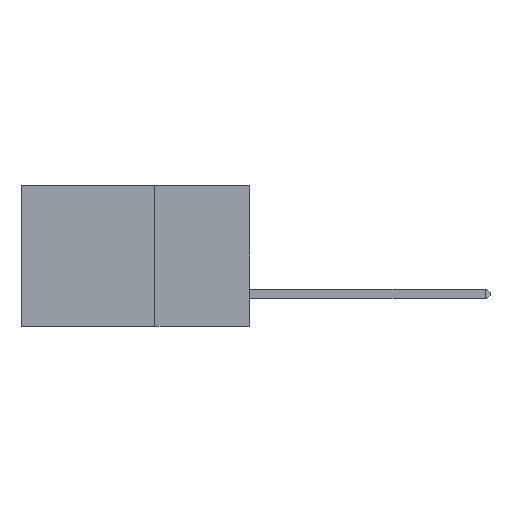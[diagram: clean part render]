
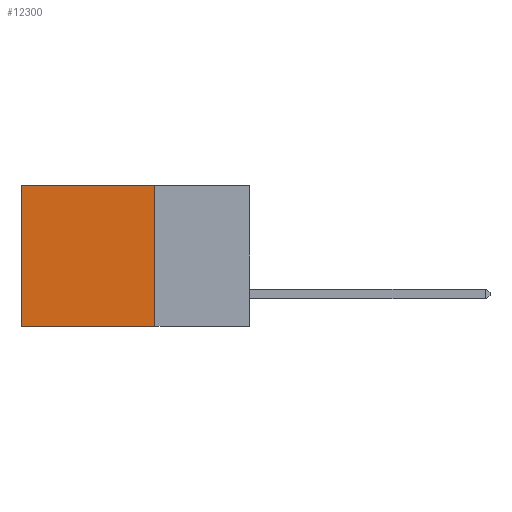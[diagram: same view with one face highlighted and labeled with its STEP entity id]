
A CAD part, left-side view. The second image highlights one B-rep face of the part: STEP entity #12300.
In plain terms, the highlighted planar face has unit normal (-1, 0, 0).
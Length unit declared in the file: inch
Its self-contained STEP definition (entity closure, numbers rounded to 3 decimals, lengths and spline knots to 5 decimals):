
#1313 = DIRECTION ( 'NONE',  ( 1., 0., 0. ) ) ;
#1460 = EDGE_CURVE ( 'NONE', #34319, #35597, #19722, .T. ) ;
#5352 = AXIS2_PLACEMENT_3D ( 'NONE', #17121, #1313, #8168 ) ;
#6060 = ORIENTED_EDGE ( 'NONE', *, *, #26684, .F. ) ;
#6569 = EDGE_CURVE ( 'NONE', #11668, #34319, #12802, .T. ) ;
#7749 = PLANE ( 'NONE',  #5352 ) ;
#8168 = DIRECTION ( 'NONE',  ( 0., 0., -1. ) ) ;
#8426 = DIRECTION ( 'NONE',  ( 0., 1., 0. ) ) ;
#8694 = CARTESIAN_POINT ( 'NONE',  ( 0.2875, 0.25, -0.37 ) ) ;
#11230 = VECTOR ( 'NONE', #17451, 39.37008 ) ;
#11352 = DIRECTION ( 'NONE',  ( 0., 0., -1. ) ) ;
#11668 = VERTEX_POINT ( 'NONE', #23386 ) ;
#12300 = ADVANCED_FACE ( 'NONE', ( #17513 ), #7749, .F. ) ;
#12786 = DIRECTION ( 'NONE',  ( 0., 1., 0. ) ) ;
#12802 = LINE ( 'NONE', #37380, #39837 ) ;
#15010 = EDGE_LOOP ( 'NONE', ( #22510, #6060, #15567, #29745 ) ) ;
#15567 = ORIENTED_EDGE ( 'NONE', *, *, #30973, .F. ) ;
#17121 = CARTESIAN_POINT ( 'NONE',  ( 0.2875, 0.25, 0. ) ) ;
#17451 = DIRECTION ( 'NONE',  ( 0., 0., -1. ) ) ;
#17513 = FACE_OUTER_BOUND ( 'NONE', #15010, .T. ) ;
#18606 = VECTOR ( 'NONE', #12786, 39.37008 ) ;
#19722 = LINE ( 'NONE', #33274, #11230 ) ;
#20080 = CARTESIAN_POINT ( 'NONE',  ( 0.2875, 0.6, -0.37 ) ) ;
#20201 = LINE ( 'NONE', #30675, #26260 ) ;
#22510 = ORIENTED_EDGE ( 'NONE', *, *, #1460, .T. ) ;
#23386 = CARTESIAN_POINT ( 'NONE',  ( 0.2875, 0.25, 0. ) ) ;
#26260 = VECTOR ( 'NONE', #11352, 39.37008 ) ;
#26684 = EDGE_CURVE ( 'NONE', #31178, #35597, #34625, .T. ) ;
#29745 = ORIENTED_EDGE ( 'NONE', *, *, #6569, .T. ) ;
#30675 = CARTESIAN_POINT ( 'NONE',  ( 0.2875, 0.25, 0. ) ) ;
#30973 = EDGE_CURVE ( 'NONE', #11668, #31178, #20201, .T. ) ;
#31178 = VERTEX_POINT ( 'NONE', #8694 ) ;
#33274 = CARTESIAN_POINT ( 'NONE',  ( 0.2875, 0.6, 0. ) ) ;
#34319 = VERTEX_POINT ( 'NONE', #36479 ) ;
#34625 = LINE ( 'NONE', #38278, #18606 ) ;
#35597 = VERTEX_POINT ( 'NONE', #20080 ) ;
#36479 = CARTESIAN_POINT ( 'NONE',  ( 0.2875, 0.6, 0. ) ) ;
#37380 = CARTESIAN_POINT ( 'NONE',  ( 0.2875, 0.25, 0. ) ) ;
#38278 = CARTESIAN_POINT ( 'NONE',  ( 0.2875, 0.25, -0.37 ) ) ;
#39837 = VECTOR ( 'NONE', #8426, 39.37008 ) ;
